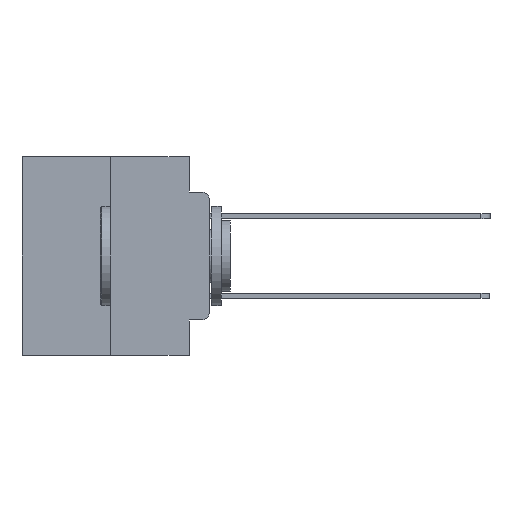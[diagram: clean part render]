
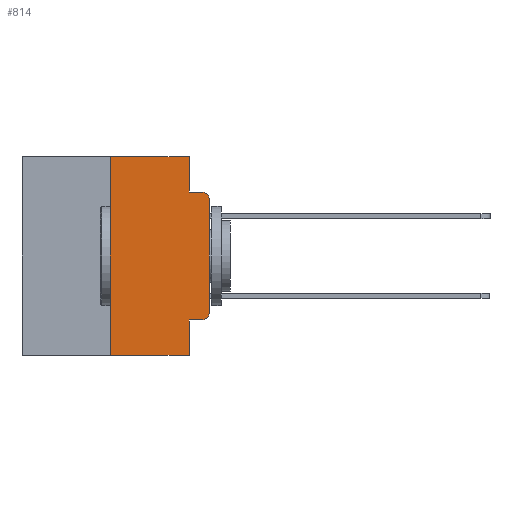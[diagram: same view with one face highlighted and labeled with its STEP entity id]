
A CAD part, left-side view. The second image highlights one B-rep face of the part: STEP entity #814.
In plain terms, the highlighted planar face has unit normal (-1, 0, 0).
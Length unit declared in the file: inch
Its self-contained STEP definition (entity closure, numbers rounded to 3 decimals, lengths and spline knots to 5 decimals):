
#611 = VECTOR ( 'NONE', #20460, 39.37008 ) ;
#814 = ADVANCED_FACE ( 'NONE', ( #10635 ), #6860, .F. ) ;
#899 = DIRECTION ( 'NONE',  ( 0., -1., 0. ) ) ;
#1139 = EDGE_CURVE ( 'NONE', #23347, #13052, #19529, .T. ) ;
#1219 = CARTESIAN_POINT ( 'NONE',  ( 0., 0.473, 0. ) ) ;
#1481 = VECTOR ( 'NONE', #7140, 39.37008 ) ;
#1706 = EDGE_CURVE ( 'NONE', #13052, #4761, #16213, .T. ) ;
#1918 = ORIENTED_EDGE ( 'NONE', *, *, #3989, .F. ) ;
#2576 = EDGE_CURVE ( 'NONE', #4761, #2584, #2686, .T. ) ;
#2584 = VERTEX_POINT ( 'NONE', #21634 ) ;
#2686 = LINE ( 'NONE', #21603, #6954 ) ;
#2822 = CARTESIAN_POINT ( 'NONE',  ( 0., 0.051, -0.4115 ) ) ;
#2969 = CARTESIAN_POINT ( 'NONE',  ( 0., 0.473, 0. ) ) ;
#3186 = VECTOR ( 'NONE', #25697, 39.37008 ) ;
#3217 = ORIENTED_EDGE ( 'NONE', *, *, #8188, .T. ) ;
#3525 = DIRECTION ( 'NONE',  ( 0., 0., -1. ) ) ;
#3989 = EDGE_CURVE ( 'NONE', #2584, #13123, #22988, .T. ) ;
#4295 = CARTESIAN_POINT ( 'NONE',  ( 0., 0., -0.1085 ) ) ;
#4761 = VERTEX_POINT ( 'NONE', #22888 ) ;
#5037 = VECTOR ( 'NONE', #899, 39.37008 ) ;
#5264 = VECTOR ( 'NONE', #12013, 39.37008 ) ;
#5464 = VERTEX_POINT ( 'NONE', #27255 ) ;
#5758 = CARTESIAN_POINT ( 'NONE',  ( 0., 0.051, -0.0885 ) ) ;
#5765 = EDGE_CURVE ( 'NONE', #23347, #25094, #13466, .T. ) ;
#6804 = EDGE_CURVE ( 'NONE', #19765, #13123, #15764, .T. ) ;
#6860 = PLANE ( 'NONE',  #22870 ) ;
#6954 = VECTOR ( 'NONE', #22144, 39.37008 ) ;
#7140 = DIRECTION ( 'NONE',  ( 0., 0., -1. ) ) ;
#7639 = AXIS2_PLACEMENT_3D ( 'NONE', #10663, #25395, #12784 ) ;
#7678 = VECTOR ( 'NONE', #22772, 39.37008 ) ;
#7749 = DIRECTION ( 'NONE',  ( 1., 0., 0. ) ) ;
#8188 = EDGE_CURVE ( 'NONE', #5464, #19765, #25541, .T. ) ;
#8237 = VERTEX_POINT ( 'NONE', #2822 ) ;
#8535 = ORIENTED_EDGE ( 'NONE', *, *, #6804, .T. ) ;
#8565 = VECTOR ( 'NONE', #24060, 39.37008 ) ;
#8596 = CARTESIAN_POINT ( 'NONE',  ( 0., 0.25, 0. ) ) ;
#9180 = CARTESIAN_POINT ( 'NONE',  ( 0., 0.02, -0.4115 ) ) ;
#10109 = DIRECTION ( 'NONE',  ( -1., 0., 0. ) ) ;
#10635 = FACE_OUTER_BOUND ( 'NONE', #21333, .T. ) ;
#10663 = CARTESIAN_POINT ( 'NONE',  ( 0., 0.02, -0.1085 ) ) ;
#11234 = AXIS2_PLACEMENT_3D ( 'NONE', #22739, #10109, #24851 ) ;
#12013 = DIRECTION ( 'NONE',  ( 0., -1., 0. ) ) ;
#12784 = DIRECTION ( 'NONE',  ( 0., 0., -1. ) ) ;
#13052 = VERTEX_POINT ( 'NONE', #8596 ) ;
#13068 = CARTESIAN_POINT ( 'NONE',  ( 0., 0., 0. ) ) ;
#13123 = VERTEX_POINT ( 'NONE', #19380 ) ;
#13298 = LINE ( 'NONE', #21768, #1481 ) ;
#13466 = LINE ( 'NONE', #13505, #8565 ) ;
#13505 = CARTESIAN_POINT ( 'NONE',  ( 0., 0.473, -0.5 ) ) ;
#15764 = CIRCLE ( 'NONE', #7639, 0.02 ) ;
#16213 = LINE ( 'NONE', #2969, #5037 ) ;
#17498 = CIRCLE ( 'NONE', #11234, 0.02 ) ;
#18856 = ORIENTED_EDGE ( 'NONE', *, *, #22824, .T. ) ;
#19380 = CARTESIAN_POINT ( 'NONE',  ( 0., 0.02, -0.0885 ) ) ;
#19529 = LINE ( 'NONE', #23671, #7678 ) ;
#19765 = VERTEX_POINT ( 'NONE', #4295 ) ;
#20229 = CARTESIAN_POINT ( 'NONE',  ( 0., 0.25, -0.5 ) ) ;
#20460 = DIRECTION ( 'NONE',  ( 0., -1., 0. ) ) ;
#21235 = ORIENTED_EDGE ( 'NONE', *, *, #24259, .T. ) ;
#21333 = EDGE_LOOP ( 'NONE', ( #3217, #8535, #1918, #26326, #27025, #22675, #22528, #21675, #21235, #18856 ) ) ;
#21603 = CARTESIAN_POINT ( 'NONE',  ( 0., 0.051, 0. ) ) ;
#21634 = CARTESIAN_POINT ( 'NONE',  ( 0., 0.051, -0.0885 ) ) ;
#21675 = ORIENTED_EDGE ( 'NONE', *, *, #27034, .F. ) ;
#21768 = CARTESIAN_POINT ( 'NONE',  ( 0., 0.051, 0. ) ) ;
#22144 = DIRECTION ( 'NONE',  ( 0., 0., -1. ) ) ;
#22528 = ORIENTED_EDGE ( 'NONE', *, *, #5765, .T. ) ;
#22675 = ORIENTED_EDGE ( 'NONE', *, *, #1139, .F. ) ;
#22739 = CARTESIAN_POINT ( 'NONE',  ( 0., 0.02, -0.3915 ) ) ;
#22772 = DIRECTION ( 'NONE',  ( 0., 0., 1. ) ) ;
#22824 = EDGE_CURVE ( 'NONE', #24025, #5464, #17498, .T. ) ;
#22870 = AXIS2_PLACEMENT_3D ( 'NONE', #1219, #7749, #3525 ) ;
#22888 = CARTESIAN_POINT ( 'NONE',  ( 0., 0.051, 0. ) ) ;
#22988 = LINE ( 'NONE', #5758, #611 ) ;
#23347 = VERTEX_POINT ( 'NONE', #20229 ) ;
#23359 = LINE ( 'NONE', #24647, #5264 ) ;
#23671 = CARTESIAN_POINT ( 'NONE',  ( 0., 0.25, 0. ) ) ;
#24025 = VERTEX_POINT ( 'NONE', #9180 ) ;
#24060 = DIRECTION ( 'NONE',  ( 0., -1., 0. ) ) ;
#24259 = EDGE_CURVE ( 'NONE', #8237, #24025, #23359, .T. ) ;
#24647 = CARTESIAN_POINT ( 'NONE',  ( 0., 0.051, -0.4115 ) ) ;
#24851 = DIRECTION ( 'NONE',  ( 0., 0., -1. ) ) ;
#25094 = VERTEX_POINT ( 'NONE', #25411 ) ;
#25395 = DIRECTION ( 'NONE',  ( -1., 0., 0. ) ) ;
#25411 = CARTESIAN_POINT ( 'NONE',  ( 0., 0.051, -0.5 ) ) ;
#25541 = LINE ( 'NONE', #13068, #3186 ) ;
#25697 = DIRECTION ( 'NONE',  ( 0., 0., 1. ) ) ;
#26326 = ORIENTED_EDGE ( 'NONE', *, *, #2576, .F. ) ;
#27025 = ORIENTED_EDGE ( 'NONE', *, *, #1706, .F. ) ;
#27034 = EDGE_CURVE ( 'NONE', #8237, #25094, #13298, .T. ) ;
#27255 = CARTESIAN_POINT ( 'NONE',  ( 0., 0., -0.3915 ) ) ;
